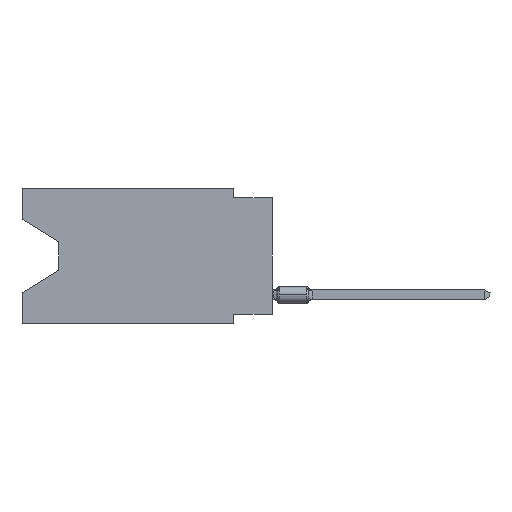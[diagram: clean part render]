
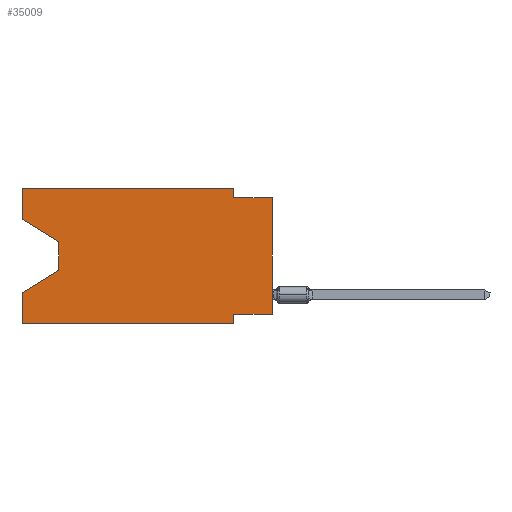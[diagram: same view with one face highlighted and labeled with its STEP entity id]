
A CAD part, left-side view. The second image highlights one B-rep face of the part: STEP entity #35009.
In plain terms, the highlighted planar face has unit normal (-1, 0, 0).
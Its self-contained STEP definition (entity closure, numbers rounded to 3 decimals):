
#967 = CARTESIAN_POINT ( 'NONE',  ( 0., 16.383, -8.89 ) ) ;
#1588 = VECTOR ( 'NONE', #4209, 1000. ) ;
#2732 = EDGE_CURVE ( 'NONE', #51438, #23224, #30573, .T. ) ;
#2790 = ORIENTED_EDGE ( 'NONE', *, *, #51750, .F. ) ;
#3589 = LINE ( 'NONE', #33021, #1588 ) ;
#3656 = VERTEX_POINT ( 'NONE', #48978 ) ;
#4209 = DIRECTION ( 'NONE',  ( 0., 0., 1. ) ) ;
#4788 = CARTESIAN_POINT ( 'NONE',  ( 0., 13.97, -3.505 ) ) ;
#4860 = CARTESIAN_POINT ( 'NONE',  ( 0., 16.383, 0. ) ) ;
#5148 = ORIENTED_EDGE ( 'NONE', *, *, #2732, .T. ) ;
#5955 = VERTEX_POINT ( 'NONE', #55499 ) ;
#6200 = VECTOR ( 'NONE', #63118, 1000. ) ;
#6582 = DIRECTION ( 'NONE',  ( 0., 0., -1. ) ) ;
#6942 = VECTOR ( 'NONE', #49596, 1000. ) ;
#8075 = EDGE_CURVE ( 'NONE', #9059, #21938, #13939, .T. ) ;
#8839 = DIRECTION ( 'NONE',  ( 0., -0.855, -0.519 ) ) ;
#9059 = VERTEX_POINT ( 'NONE', #41200 ) ;
#12063 = CARTESIAN_POINT ( 'NONE',  ( 0., 2.54, -0.635 ) ) ;
#12505 = DIRECTION ( 'NONE',  ( 0., 0.855, -0.519 ) ) ;
#12741 = ORIENTED_EDGE ( 'NONE', *, *, #52624, .F. ) ;
#13819 = EDGE_CURVE ( 'NONE', #46310, #46188, #15967, .T. ) ;
#13939 = LINE ( 'NONE', #62613, #24904 ) ;
#14757 = VERTEX_POINT ( 'NONE', #34794 ) ;
#15156 = DIRECTION ( 'NONE',  ( 0., 0., -1. ) ) ;
#15608 = LINE ( 'NONE', #61973, #20234 ) ;
#15967 = LINE ( 'NONE', #21964, #6942 ) ;
#16622 = EDGE_CURVE ( 'NONE', #21938, #3656, #24639, .T. ) ;
#17934 = LINE ( 'NONE', #56366, #46309 ) ;
#19183 = EDGE_CURVE ( 'NONE', #3656, #14757, #17934, .T. ) ;
#20234 = VECTOR ( 'NONE', #23846, 1000. ) ;
#20414 = EDGE_LOOP ( 'NONE', ( #43615, #28569, #35238, #43405, #5148, #2790, #20448, #36162, #56514, #12741, #58601, #48287 ) ) ;
#20448 = ORIENTED_EDGE ( 'NONE', *, *, #51945, .F. ) ;
#20638 = CARTESIAN_POINT ( 'NONE',  ( 0., 2.54, 0. ) ) ;
#21227 = LINE ( 'NONE', #35955, #62057 ) ;
#21824 = DIRECTION ( 'NONE',  ( 0., -1., 0. ) ) ;
#21938 = VERTEX_POINT ( 'NONE', #4788 ) ;
#21964 = CARTESIAN_POINT ( 'NONE',  ( 0., 0., -0.635 ) ) ;
#22957 = PLANE ( 'NONE',  #60834 ) ;
#23224 = VERTEX_POINT ( 'NONE', #60464 ) ;
#23846 = DIRECTION ( 'NONE',  ( 0., 0., 1. ) ) ;
#24639 = LINE ( 'NONE', #43589, #6200 ) ;
#24820 = DIRECTION ( 'NONE',  ( 0., 0., -1. ) ) ;
#24904 = VECTOR ( 'NONE', #8839, 1000. ) ;
#24955 = VECTOR ( 'NONE', #6582, 1000. ) ;
#26079 = VECTOR ( 'NONE', #21824, 1000. ) ;
#27277 = LINE ( 'NONE', #35934, #26079 ) ;
#28569 = ORIENTED_EDGE ( 'NONE', *, *, #16622, .T. ) ;
#28801 = EDGE_CURVE ( 'NONE', #51438, #14757, #15608, .T. ) ;
#30573 = LINE ( 'NONE', #50091, #49866 ) ;
#33021 = CARTESIAN_POINT ( 'NONE',  ( 0., 0., 0. ) ) ;
#33134 = LINE ( 'NONE', #57459, #59073 ) ;
#33520 = LINE ( 'NONE', #38643, #55002 ) ;
#34794 = CARTESIAN_POINT ( 'NONE',  ( 0., 16.383, -6.852 ) ) ;
#34871 = VERTEX_POINT ( 'NONE', #60766 ) ;
#35009 = ADVANCED_FACE ( 'NONE', ( #59036 ), #22957, .F. ) ;
#35238 = ORIENTED_EDGE ( 'NONE', *, *, #19183, .T. ) ;
#35934 = CARTESIAN_POINT ( 'NONE',  ( 0., 16.383, 0. ) ) ;
#35955 = CARTESIAN_POINT ( 'NONE',  ( 0., 16.383, 0. ) ) ;
#36162 = ORIENTED_EDGE ( 'NONE', *, *, #55037, .T. ) ;
#38643 = CARTESIAN_POINT ( 'NONE',  ( 0., 2.54, -8.89 ) ) ;
#41200 = CARTESIAN_POINT ( 'NONE',  ( 0., 16.383, -2.038 ) ) ;
#43133 = DIRECTION ( 'NONE',  ( 1., 0., 0. ) ) ;
#43405 = ORIENTED_EDGE ( 'NONE', *, *, #28801, .F. ) ;
#43589 = CARTESIAN_POINT ( 'NONE',  ( 0., 13.97, -3.505 ) ) ;
#43615 = ORIENTED_EDGE ( 'NONE', *, *, #8075, .T. ) ;
#45363 = CARTESIAN_POINT ( 'NONE',  ( 0., 0., -0.635 ) ) ;
#45893 = DIRECTION ( 'NONE',  ( 0., 0., 1. ) ) ;
#46188 = VERTEX_POINT ( 'NONE', #45363 ) ;
#46309 = VECTOR ( 'NONE', #12505, 1000. ) ;
#46310 = VERTEX_POINT ( 'NONE', #12063 ) ;
#46993 = CARTESIAN_POINT ( 'NONE',  ( 0., 16.383, 0. ) ) ;
#48287 = ORIENTED_EDGE ( 'NONE', *, *, #50011, .F. ) ;
#48381 = CARTESIAN_POINT ( 'NONE',  ( 0., 0., -8.255 ) ) ;
#48978 = CARTESIAN_POINT ( 'NONE',  ( 0., 13.97, -5.385 ) ) ;
#49596 = DIRECTION ( 'NONE',  ( 0., -1., 0. ) ) ;
#49866 = VECTOR ( 'NONE', #61594, 1000. ) ;
#50011 = EDGE_CURVE ( 'NONE', #9059, #62107, #21227, .T. ) ;
#50091 = CARTESIAN_POINT ( 'NONE',  ( 0., 16.383, -8.89 ) ) ;
#50434 = LINE ( 'NONE', #20638, #24955 ) ;
#51438 = VERTEX_POINT ( 'NONE', #967 ) ;
#51719 = DIRECTION ( 'NONE',  ( 0., 1., 0. ) ) ;
#51750 = EDGE_CURVE ( 'NONE', #34871, #23224, #33520, .T. ) ;
#51945 = EDGE_CURVE ( 'NONE', #55038, #34871, #33134, .T. ) ;
#52624 = EDGE_CURVE ( 'NONE', #5955, #46310, #50434, .T. ) ;
#55002 = VECTOR ( 'NONE', #24820, 1000. ) ;
#55037 = EDGE_CURVE ( 'NONE', #55038, #46188, #3589, .T. ) ;
#55038 = VERTEX_POINT ( 'NONE', #48381 ) ;
#55499 = CARTESIAN_POINT ( 'NONE',  ( 0., 2.54, 0. ) ) ;
#56366 = CARTESIAN_POINT ( 'NONE',  ( 0., 13.97, -5.385 ) ) ;
#56514 = ORIENTED_EDGE ( 'NONE', *, *, #13819, .F. ) ;
#57459 = CARTESIAN_POINT ( 'NONE',  ( 0., 0., -8.255 ) ) ;
#57627 = EDGE_CURVE ( 'NONE', #62107, #5955, #27277, .T. ) ;
#58601 = ORIENTED_EDGE ( 'NONE', *, *, #57627, .F. ) ;
#59036 = FACE_OUTER_BOUND ( 'NONE', #20414, .T. ) ;
#59073 = VECTOR ( 'NONE', #51719, 1000. ) ;
#60464 = CARTESIAN_POINT ( 'NONE',  ( 0., 2.54, -8.89 ) ) ;
#60766 = CARTESIAN_POINT ( 'NONE',  ( 0., 2.54, -8.255 ) ) ;
#60834 = AXIS2_PLACEMENT_3D ( 'NONE', #46993, #43133, #15156 ) ;
#61594 = DIRECTION ( 'NONE',  ( 0., -1., 0. ) ) ;
#61973 = CARTESIAN_POINT ( 'NONE',  ( 0., 16.383, 0. ) ) ;
#62057 = VECTOR ( 'NONE', #45893, 1000. ) ;
#62107 = VERTEX_POINT ( 'NONE', #4860 ) ;
#62613 = CARTESIAN_POINT ( 'NONE',  ( 0., 16.383, -2.038 ) ) ;
#63118 = DIRECTION ( 'NONE',  ( 0., 0., -1. ) ) ;
